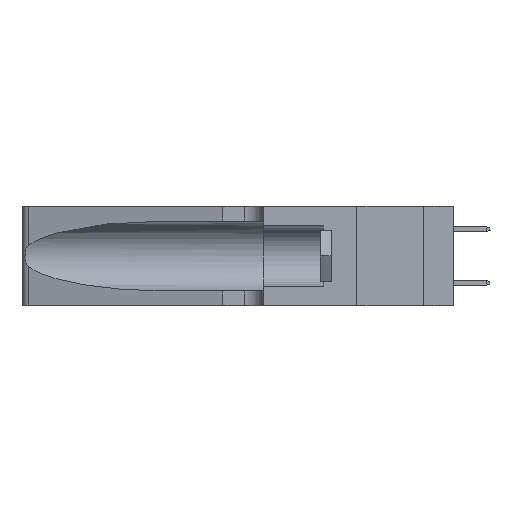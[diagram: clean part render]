
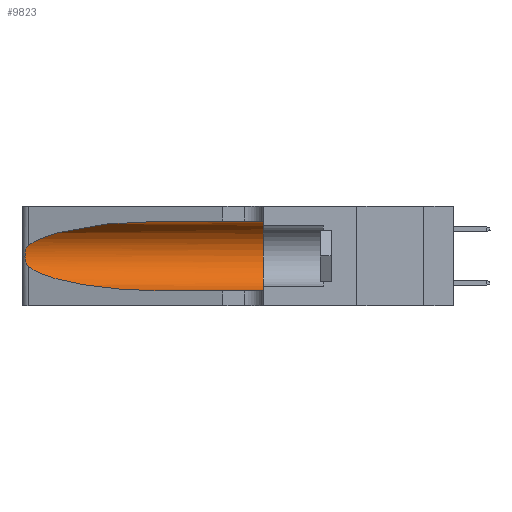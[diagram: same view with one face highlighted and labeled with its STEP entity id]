
A CAD part, left-side view. The second image highlights one B-rep face of the part: STEP entity #9823.
In plain terms, the highlighted cylindrical face has radius 3.308 mm (diameter 6.617 mm), a partial arc.
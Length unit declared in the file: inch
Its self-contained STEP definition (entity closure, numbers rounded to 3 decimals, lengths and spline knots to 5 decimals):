
#671 = CYLINDRICAL_SURFACE ( 'NONE', #22611, 0.13025 ) ;
#2857 = DIRECTION ( 'NONE',  ( 0., 0., -1. ) ) ;
#4354 = CARTESIAN_POINT ( 'NONE',  ( 0.18966, 0.96281, 0.05475 ) ) ;
#5499 = CARTESIAN_POINT ( 'NONE',  ( 0.26017, 1.23833, 0.17102 ) ) ;
#5954 = LINE ( 'NONE', #27983, #39019 ) ;
#6093 = B_SPLINE_CURVE_WITH_KNOTS ( 'NONE', 3,
 ( #37690, #8693, #38096, #22032, #8270, #37473, #28156, #34515, #5499, #34083, #18431, #31318, #30922, #34919 ),
 .UNSPECIFIED., .F., .F.,
 ( 4, 2, 2, 2, 2, 2, 4 ),
 ( 0., 0.00027, 0.00053, 0.00107, 0.0016, 0.00187, 0.00214 ),
 .UNSPECIFIED. ) ;
#6407 =( BOUNDED_CURVE ( )  B_SPLINE_CURVE ( 3, ( #27249, #33366, #4354, #30193 ),
 .UNSPECIFIED., .F., .F. ) 
 B_SPLINE_CURVE_WITH_KNOTS ( ( 4, 4 ),
 ( 3.44316, 4.71239 ),
 .UNSPECIFIED. ) 
 CURVE ( )  GEOMETRIC_REPRESENTATION_ITEM ( )  RATIONAL_B_SPLINE_CURVE ( ( 1., 0.87, 0.87, 1. ) ) 
 REPRESENTATION_ITEM ( '' )  );
#8270 = CARTESIAN_POINT ( 'NONE',  ( 0.25854, 1.2359, 0.20912 ) ) ;
#8323 = VERTEX_POINT ( 'NONE', #12987 ) ;
#8693 = CARTESIAN_POINT ( 'NONE',  ( 0.25555, 1.22994, 0.2215 ) ) ;
#8786 = ORIENTED_EDGE ( 'NONE', *, *, #26948, .T. ) ;
#9823 = ADVANCED_FACE ( 'NONE', ( #16586 ), #671, .F. ) ;
#12987 = CARTESIAN_POINT ( 'NONE',  ( 0.1305, 0.72297, 0.31525 ) ) ;
#13624 = CARTESIAN_POINT ( 'NONE',  ( 0.1305, 1.61858, 0.185 ) ) ;
#15422 = EDGE_LOOP ( 'NONE', ( #20470, #35121, #38446, #8786, #39875, #22825 ) ) ;
#15548 = CARTESIAN_POINT ( 'NONE',  ( 0.2373, 1.15595, 0.28018 ) ) ;
#16586 = FACE_OUTER_BOUND ( 'NONE', #15422, .T. ) ;
#17186 = AXIS2_PLACEMENT_3D ( 'NONE', #39548, #20554, #20346 ) ;
#17264 = CARTESIAN_POINT ( 'NONE',  ( 0.1305, 0.72297, 0.31525 ) ) ;
#18060 =( BOUNDED_CURVE ( )  B_SPLINE_CURVE ( 3, ( #17264, #30169, #15548, #18101 ),
 .UNSPECIFIED., .F., .F. ) 
 B_SPLINE_CURVE_WITH_KNOTS ( ( 4, 4 ),
 ( 1.5708, 2.84003 ),
 .UNSPECIFIED. ) 
 CURVE ( )  GEOMETRIC_REPRESENTATION_ITEM ( )  RATIONAL_B_SPLINE_CURVE ( ( 1., 0.87, 0.87, 1. ) ) 
 REPRESENTATION_ITEM ( '' )  );
#18101 = CARTESIAN_POINT ( 'NONE',  ( 0.25487, 1.22718, 0.22369 ) ) ;
#18431 = CARTESIAN_POINT ( 'NONE',  ( 0.25789, 1.23486, 0.15765 ) ) ;
#19390 = DIRECTION ( 'NONE',  ( 0., -1., 0. ) ) ;
#20346 = DIRECTION ( 'NONE',  ( 0., 0., 1. ) ) ;
#20470 = ORIENTED_EDGE ( 'NONE', *, *, #26412, .T. ) ;
#20554 = DIRECTION ( 'NONE',  ( 0., 1., 0. ) ) ;
#20967 = VECTOR ( 'NONE', #19390, 39.37008 ) ;
#21734 = CARTESIAN_POINT ( 'NONE',  ( 0.1305, 1.61858, 0.31525 ) ) ;
#21874 = EDGE_CURVE ( 'NONE', #8323, #32168, #22151, .T. ) ;
#22032 = CARTESIAN_POINT ( 'NONE',  ( 0.25787, 1.23484, 0.2124 ) ) ;
#22151 = LINE ( 'NONE', #21734, #20967 ) ;
#22611 = AXIS2_PLACEMENT_3D ( 'NONE', #13624, #23355, #2857 ) ;
#22825 = ORIENTED_EDGE ( 'NONE', *, *, #21874, .F. ) ;
#23355 = DIRECTION ( 'NONE',  ( 0., -1., 0. ) ) ;
#25907 = CARTESIAN_POINT ( 'NONE',  ( 0.25487, 1.22718, 0.14631 ) ) ;
#26412 = EDGE_CURVE ( 'NONE', #8323, #31109, #18060, .T. ) ;
#26910 = CARTESIAN_POINT ( 'NONE',  ( 0.1305, 0.35, 0.05475 ) ) ;
#26948 = EDGE_CURVE ( 'NONE', #31283, #37058, #5954, .T. ) ;
#27249 = CARTESIAN_POINT ( 'NONE',  ( 0.25487, 1.22718, 0.14631 ) ) ;
#27948 = VERTEX_POINT ( 'NONE', #25907 ) ;
#27983 = CARTESIAN_POINT ( 'NONE',  ( 0.1305, 1.61858, 0.05475 ) ) ;
#27985 = CIRCLE ( 'NONE', #17186, 0.13025 ) ;
#28156 = CARTESIAN_POINT ( 'NONE',  ( 0.26075, 1.23896, 0.19203 ) ) ;
#28738 = EDGE_CURVE ( 'NONE', #31109, #27948, #6093, .T. ) ;
#29487 = EDGE_CURVE ( 'NONE', #27948, #31283, #6407, .T. ) ;
#29748 = CARTESIAN_POINT ( 'NONE',  ( 0.1305, 0.72297, 0.05475 ) ) ;
#30169 = CARTESIAN_POINT ( 'NONE',  ( 0.18966, 0.96281, 0.31525 ) ) ;
#30193 = CARTESIAN_POINT ( 'NONE',  ( 0.1305, 0.72297, 0.05475 ) ) ;
#30922 = CARTESIAN_POINT ( 'NONE',  ( 0.25555, 1.22993, 0.14849 ) ) ;
#31109 = VERTEX_POINT ( 'NONE', #31860 ) ;
#31283 = VERTEX_POINT ( 'NONE', #29748 ) ;
#31318 = CARTESIAN_POINT ( 'NONE',  ( 0.25639, 1.23186, 0.15144 ) ) ;
#31860 = CARTESIAN_POINT ( 'NONE',  ( 0.25487, 1.22718, 0.22369 ) ) ;
#32168 = VERTEX_POINT ( 'NONE', #36007 ) ;
#33366 = CARTESIAN_POINT ( 'NONE',  ( 0.2373, 1.15595, 0.08982 ) ) ;
#34083 = CARTESIAN_POINT ( 'NONE',  ( 0.25856, 1.23593, 0.16098 ) ) ;
#34515 = CARTESIAN_POINT ( 'NONE',  ( 0.26075, 1.23896, 0.178 ) ) ;
#34919 = CARTESIAN_POINT ( 'NONE',  ( 0.25487, 1.22718, 0.14631 ) ) ;
#35121 = ORIENTED_EDGE ( 'NONE', *, *, #28738, .T. ) ;
#36007 = CARTESIAN_POINT ( 'NONE',  ( 0.1305, 0.35, 0.31525 ) ) ;
#37058 = VERTEX_POINT ( 'NONE', #26910 ) ;
#37309 = DIRECTION ( 'NONE',  ( 0., -1., 0. ) ) ;
#37473 = CARTESIAN_POINT ( 'NONE',  ( 0.26018, 1.23835, 0.19895 ) ) ;
#37690 = CARTESIAN_POINT ( 'NONE',  ( 0.25487, 1.22718, 0.22369 ) ) ;
#38096 = CARTESIAN_POINT ( 'NONE',  ( 0.25639, 1.23184, 0.21858 ) ) ;
#38148 = EDGE_CURVE ( 'NONE', #32168, #37058, #27985, .T. ) ;
#38446 = ORIENTED_EDGE ( 'NONE', *, *, #29487, .T. ) ;
#39019 = VECTOR ( 'NONE', #37309, 39.37008 ) ;
#39548 = CARTESIAN_POINT ( 'NONE',  ( 0.1305, 0.35, 0.185 ) ) ;
#39875 = ORIENTED_EDGE ( 'NONE', *, *, #38148, .F. ) ;
